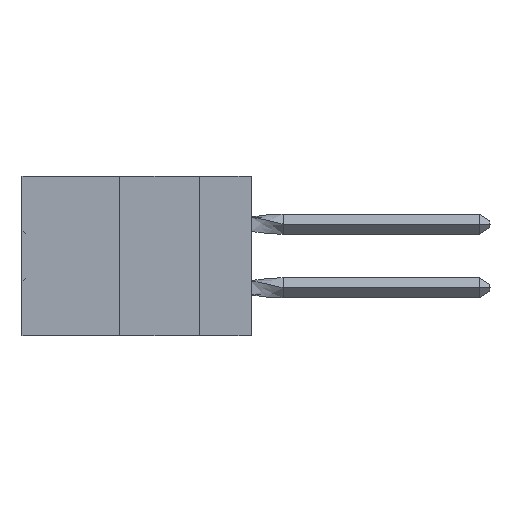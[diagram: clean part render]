
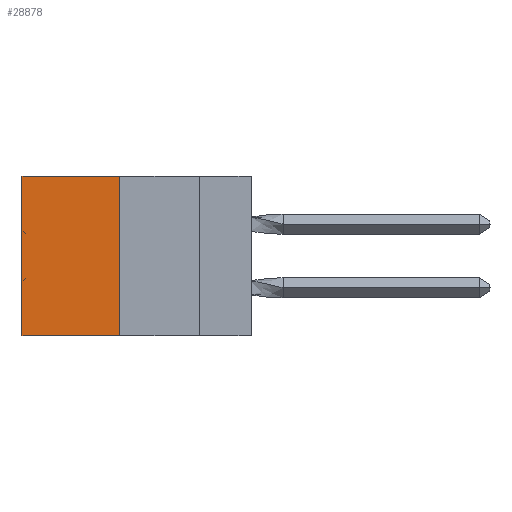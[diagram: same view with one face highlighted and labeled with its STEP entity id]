
A CAD part, left-side view. The second image highlights one B-rep face of the part: STEP entity #28878.
In plain terms, the highlighted planar face has unit normal (-1, 0, 0).
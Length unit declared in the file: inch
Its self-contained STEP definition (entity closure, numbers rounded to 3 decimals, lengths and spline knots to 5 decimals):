
#6126 = CARTESIAN_POINT ( 'NONE',  ( 0.305, 0.72, 0. ) ) ;
#6526 = EDGE_CURVE ( 'NONE', #54378, #26428, #30156, .T. ) ;
#10028 = EDGE_CURVE ( 'NONE', #32214, #27315, #51841, .T. ) ;
#11753 = DIRECTION ( 'NONE',  ( 0., 1., 0. ) ) ;
#12013 = CARTESIAN_POINT ( 'NONE',  ( 0.305, 0.413, -0.5 ) ) ;
#12411 = DIRECTION ( 'NONE',  ( 1., 0., 0. ) ) ;
#13418 = FACE_OUTER_BOUND ( 'NONE', #34820, .T. ) ;
#17895 = DIRECTION ( 'NONE',  ( 0., 0., -1. ) ) ;
#19316 = VECTOR ( 'NONE', #42110, 39.37008 ) ;
#20634 = EDGE_CURVE ( 'NONE', #54378, #32214, #58400, .T. ) ;
#20706 = LINE ( 'NONE', #45519, #30976 ) ;
#26428 = VERTEX_POINT ( 'NONE', #29985 ) ;
#26566 = PLANE ( 'NONE',  #50828 ) ;
#27315 = VERTEX_POINT ( 'NONE', #35836 ) ;
#27530 = ORIENTED_EDGE ( 'NONE', *, *, #43547, .F. ) ;
#28878 = ADVANCED_FACE ( 'NONE', ( #13418 ), #26566, .F. ) ;
#29985 = CARTESIAN_POINT ( 'NONE',  ( 0.305, 0.413, -0.5 ) ) ;
#30156 = LINE ( 'NONE', #32251, #52264 ) ;
#30976 = VECTOR ( 'NONE', #11753, 39.37008 ) ;
#32214 = VERTEX_POINT ( 'NONE', #6126 ) ;
#32251 = CARTESIAN_POINT ( 'NONE',  ( 0.305, 0.413, -0.5 ) ) ;
#33356 = DIRECTION ( 'NONE',  ( 0., 0., -1. ) ) ;
#34820 = EDGE_LOOP ( 'NONE', ( #58312, #27530, #53637, #59234 ) ) ;
#35836 = CARTESIAN_POINT ( 'NONE',  ( 0.305, 0.72, -0.5 ) ) ;
#39734 = CARTESIAN_POINT ( 'NONE',  ( 0.305, 0.413, 0. ) ) ;
#42110 = DIRECTION ( 'NONE',  ( 0., 1., 0. ) ) ;
#42889 = CARTESIAN_POINT ( 'NONE',  ( 0.305, 0.72, -0.5 ) ) ;
#43547 = EDGE_CURVE ( 'NONE', #26428, #27315, #20706, .T. ) ;
#45519 = CARTESIAN_POINT ( 'NONE',  ( 0.305, 0.413, -0.5 ) ) ;
#46492 = CARTESIAN_POINT ( 'NONE',  ( 0.305, 0.413, 0. ) ) ;
#46736 = VECTOR ( 'NONE', #33356, 39.37008 ) ;
#50828 = AXIS2_PLACEMENT_3D ( 'NONE', #12013, #12411, #59142 ) ;
#51841 = LINE ( 'NONE', #42889, #46736 ) ;
#52264 = VECTOR ( 'NONE', #17895, 39.37008 ) ;
#53637 = ORIENTED_EDGE ( 'NONE', *, *, #6526, .F. ) ;
#54378 = VERTEX_POINT ( 'NONE', #39734 ) ;
#58312 = ORIENTED_EDGE ( 'NONE', *, *, #10028, .T. ) ;
#58400 = LINE ( 'NONE', #46492, #19316 ) ;
#59142 = DIRECTION ( 'NONE',  ( 0., 0., -1. ) ) ;
#59234 = ORIENTED_EDGE ( 'NONE', *, *, #20634, .T. ) ;
